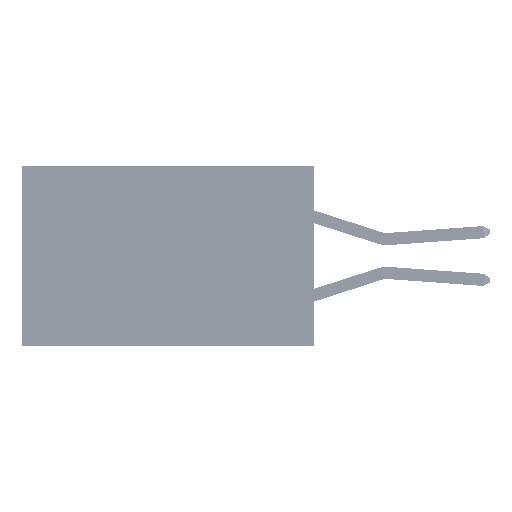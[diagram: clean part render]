
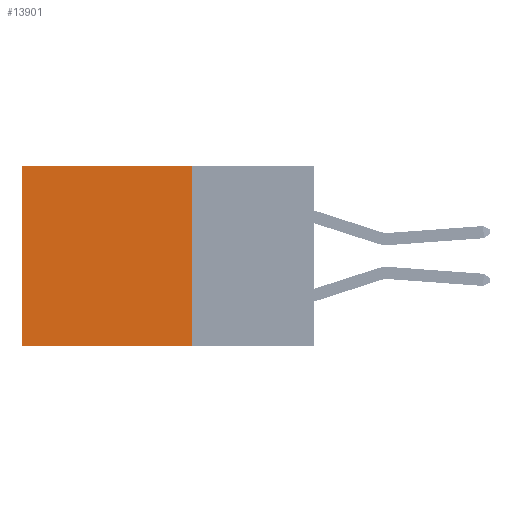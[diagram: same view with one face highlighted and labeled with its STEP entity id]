
A CAD part, left-side view. The second image highlights one B-rep face of the part: STEP entity #13901.
In plain terms, the highlighted planar face has unit normal (-1, 0, 0).
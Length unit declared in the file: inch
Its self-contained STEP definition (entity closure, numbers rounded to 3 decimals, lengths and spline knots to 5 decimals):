
#247 = EDGE_CURVE ( 'NONE', #12673, #37562, #33920, .T. ) ;
#3798 = ORIENTED_EDGE ( 'NONE', *, *, #16526, .T. ) ;
#4635 = PLANE ( 'NONE',  #18587 ) ;
#5113 = DIRECTION ( 'NONE',  ( 0., 1., 0. ) ) ;
#11791 = DIRECTION ( 'NONE',  ( 0., 1., 0. ) ) ;
#12673 = VERTEX_POINT ( 'NONE', #22020 ) ;
#12782 = FACE_OUTER_BOUND ( 'NONE', #25941, .T. ) ;
#13048 = CARTESIAN_POINT ( 'NONE',  ( 0.2875, 0.6, 0. ) ) ;
#13568 = VECTOR ( 'NONE', #5113, 39.37008 ) ;
#13901 = ADVANCED_FACE ( 'NONE', ( #12782 ), #4635, .F. ) ;
#15507 = VERTEX_POINT ( 'NONE', #45430 ) ;
#16526 = EDGE_CURVE ( 'NONE', #38694, #15507, #33797, .T. ) ;
#18116 = DIRECTION ( 'NONE',  ( 0., 0., -1. ) ) ;
#18587 = AXIS2_PLACEMENT_3D ( 'NONE', #43920, #36223, #20417 ) ;
#18857 = CARTESIAN_POINT ( 'NONE',  ( 0.2875, 0.25, -0.37 ) ) ;
#19421 = CARTESIAN_POINT ( 'NONE',  ( 0.2875, 0.25, 0. ) ) ;
#20417 = DIRECTION ( 'NONE',  ( 0., 0., -1. ) ) ;
#22020 = CARTESIAN_POINT ( 'NONE',  ( 0.2875, 0.25, 0. ) ) ;
#23743 = CARTESIAN_POINT ( 'NONE',  ( 0.2875, 0.25, -0.37 ) ) ;
#25941 = EDGE_LOOP ( 'NONE', ( #3798, #47609, #45653, #31647 ) ) ;
#28306 = EDGE_CURVE ( 'NONE', #12673, #38694, #31866, .T. ) ;
#31647 = ORIENTED_EDGE ( 'NONE', *, *, #28306, .T. ) ;
#31866 = LINE ( 'NONE', #19421, #42541 ) ;
#33570 = EDGE_CURVE ( 'NONE', #37562, #15507, #39063, .T. ) ;
#33797 = LINE ( 'NONE', #37631, #41569 ) ;
#33920 = LINE ( 'NONE', #48498, #42727 ) ;
#34561 = DIRECTION ( 'NONE',  ( 0., 0., -1. ) ) ;
#36223 = DIRECTION ( 'NONE',  ( 1., 0., 0. ) ) ;
#37562 = VERTEX_POINT ( 'NONE', #18857 ) ;
#37631 = CARTESIAN_POINT ( 'NONE',  ( 0.2875, 0.6, 0. ) ) ;
#38694 = VERTEX_POINT ( 'NONE', #13048 ) ;
#39063 = LINE ( 'NONE', #23743, #13568 ) ;
#41569 = VECTOR ( 'NONE', #34561, 39.37008 ) ;
#42541 = VECTOR ( 'NONE', #11791, 39.37008 ) ;
#42727 = VECTOR ( 'NONE', #18116, 39.37008 ) ;
#43920 = CARTESIAN_POINT ( 'NONE',  ( 0.2875, 0.25, 0. ) ) ;
#45430 = CARTESIAN_POINT ( 'NONE',  ( 0.2875, 0.6, -0.37 ) ) ;
#45653 = ORIENTED_EDGE ( 'NONE', *, *, #247, .F. ) ;
#47609 = ORIENTED_EDGE ( 'NONE', *, *, #33570, .F. ) ;
#48498 = CARTESIAN_POINT ( 'NONE',  ( 0.2875, 0.25, 0. ) ) ;
